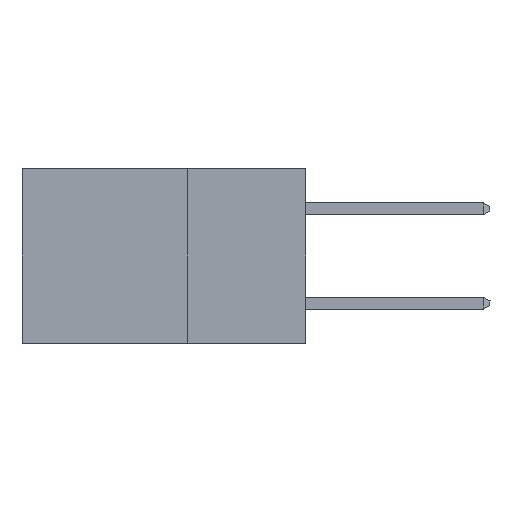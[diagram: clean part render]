
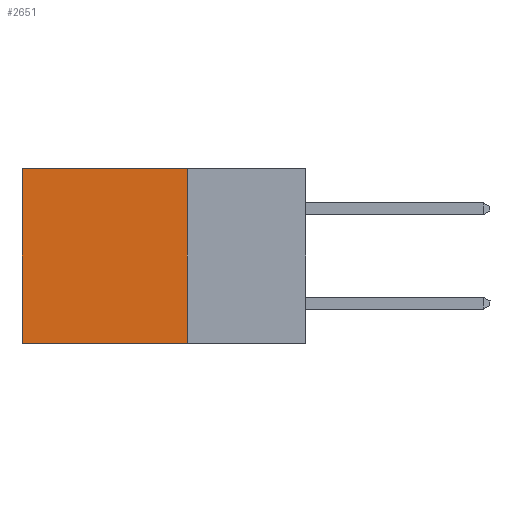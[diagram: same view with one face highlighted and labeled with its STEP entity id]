
A CAD part, left-side view. The second image highlights one B-rep face of the part: STEP entity #2651.
In plain terms, the highlighted planar face has unit normal (-1, 0, 0).
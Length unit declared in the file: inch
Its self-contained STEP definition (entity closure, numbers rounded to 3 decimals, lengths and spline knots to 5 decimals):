
#68 = VERTEX_POINT ( 'NONE', #10797 ) ;
#502 = CARTESIAN_POINT ( 'NONE',  ( 0.298, 0.25, -0.37 ) ) ;
#942 = VERTEX_POINT ( 'NONE', #1504 ) ;
#1016 = VERTEX_POINT ( 'NONE', #502 ) ;
#1073 = VECTOR ( 'NONE', #1877, 39.37008 ) ;
#1250 = VECTOR ( 'NONE', #7666, 39.37008 ) ;
#1504 = CARTESIAN_POINT ( 'NONE',  ( 0.298, 0.6, 0. ) ) ;
#1785 = CARTESIAN_POINT ( 'NONE',  ( 0.298, 0.25, -0.37 ) ) ;
#1877 = DIRECTION ( 'NONE',  ( 0., 0., -1. ) ) ;
#2185 = CARTESIAN_POINT ( 'NONE',  ( 0.298, 0.25, 0. ) ) ;
#2540 = EDGE_CURVE ( 'NONE', #68, #1016, #10336, .T. ) ;
#2651 = ADVANCED_FACE ( 'NONE', ( #5809 ), #9524, .F. ) ;
#2878 = ORIENTED_EDGE ( 'NONE', *, *, #13216, .F. ) ;
#2893 = DIRECTION ( 'NONE',  ( 0., 1., 0. ) ) ;
#3033 = ORIENTED_EDGE ( 'NONE', *, *, #2540, .F. ) ;
#3736 = CARTESIAN_POINT ( 'NONE',  ( 0.298, 0.25, 0. ) ) ;
#4274 = VECTOR ( 'NONE', #10115, 39.37008 ) ;
#4629 = EDGE_CURVE ( 'NONE', #942, #6733, #12472, .T. ) ;
#5809 = FACE_OUTER_BOUND ( 'NONE', #10055, .T. ) ;
#5920 = EDGE_CURVE ( 'NONE', #68, #942, #10127, .T. ) ;
#6733 = VERTEX_POINT ( 'NONE', #7234 ) ;
#7234 = CARTESIAN_POINT ( 'NONE',  ( 0.298, 0.6, -0.37 ) ) ;
#7339 = DIRECTION ( 'NONE',  ( 1., 0., 0. ) ) ;
#7480 = DIRECTION ( 'NONE',  ( 0., 0., -1. ) ) ;
#7666 = DIRECTION ( 'NONE',  ( 0., 1., 0. ) ) ;
#7758 = AXIS2_PLACEMENT_3D ( 'NONE', #2185, #7339, #7480 ) ;
#7936 = ORIENTED_EDGE ( 'NONE', *, *, #4629, .T. ) ;
#8391 = CARTESIAN_POINT ( 'NONE',  ( 0.298, 0.6, 0. ) ) ;
#9524 = PLANE ( 'NONE',  #7758 ) ;
#10055 = EDGE_LOOP ( 'NONE', ( #7936, #2878, #3033, #12821 ) ) ;
#10115 = DIRECTION ( 'NONE',  ( 0., 0., -1. ) ) ;
#10127 = LINE ( 'NONE', #11001, #1250 ) ;
#10336 = LINE ( 'NONE', #3736, #4274 ) ;
#10797 = CARTESIAN_POINT ( 'NONE',  ( 0.298, 0.25, 0. ) ) ;
#11001 = CARTESIAN_POINT ( 'NONE',  ( 0.298, 0.25, 0. ) ) ;
#11056 = VECTOR ( 'NONE', #2893, 39.37008 ) ;
#12472 = LINE ( 'NONE', #8391, #1073 ) ;
#12821 = ORIENTED_EDGE ( 'NONE', *, *, #5920, .T. ) ;
#13216 = EDGE_CURVE ( 'NONE', #1016, #6733, #13755, .T. ) ;
#13755 = LINE ( 'NONE', #1785, #11056 ) ;
